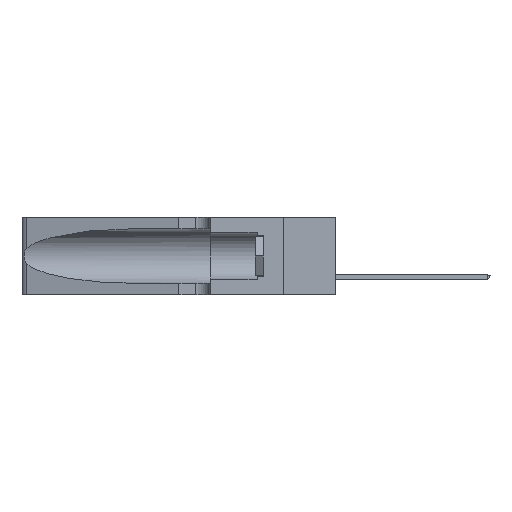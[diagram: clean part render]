
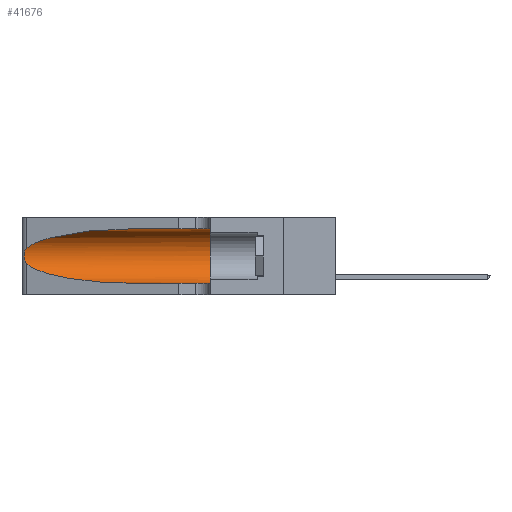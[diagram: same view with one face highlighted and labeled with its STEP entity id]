
A CAD part, left-side view. The second image highlights one B-rep face of the part: STEP entity #41676.
In plain terms, the highlighted cylindrical face has radius 3.308 mm (diameter 6.617 mm), a partial arc.
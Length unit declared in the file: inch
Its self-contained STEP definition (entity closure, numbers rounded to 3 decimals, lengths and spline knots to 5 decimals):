
#267 = EDGE_CURVE ( 'NONE', #30644, #3857, #19084, .T. ) ;
#515 = DIRECTION ( 'NONE',  ( 0., -1., 0. ) ) ;
#668 = VERTEX_POINT ( 'NONE', #48309 ) ;
#839 = FACE_OUTER_BOUND ( 'NONE', #32992, .T. ) ;
#2141 = CARTESIAN_POINT ( 'NONE',  ( 0.25487, 1.22718, 0.22369 ) ) ;
#3857 = VERTEX_POINT ( 'NONE', #40287 ) ;
#4057 = CARTESIAN_POINT ( 'NONE',  ( 0.25639, 1.23186, 0.15144 ) ) ;
#4203 = CARTESIAN_POINT ( 'NONE',  ( 0.1305, 1.61858, 0.31525 ) ) ;
#6728 = CARTESIAN_POINT ( 'NONE',  ( 0.25487, 1.22718, 0.14631 ) ) ;
#7945 = ORIENTED_EDGE ( 'NONE', *, *, #267, .F. ) ;
#7976 = CARTESIAN_POINT ( 'NONE',  ( 0.25487, 1.22718, 0.14631 ) ) ;
#9112 = VECTOR ( 'NONE', #19098, 39.37008 ) ;
#9765 = VERTEX_POINT ( 'NONE', #10908 ) ;
#10325 = AXIS2_PLACEMENT_3D ( 'NONE', #36463, #41348, #26176 ) ;
#10908 = CARTESIAN_POINT ( 'NONE',  ( 0.1305, 0.72297, 0.05475 ) ) ;
#11114 = ORIENTED_EDGE ( 'NONE', *, *, #35171, .F. ) ;
#11608 = CARTESIAN_POINT ( 'NONE',  ( 0.25555, 1.22993, 0.14849 ) ) ;
#11765 = VERTEX_POINT ( 'NONE', #6728 ) ;
#12239 = CARTESIAN_POINT ( 'NONE',  ( 0.1305, 1.61858, 0.05475 ) ) ;
#14107 =( BOUNDED_CURVE ( )  B_SPLINE_CURVE ( 3, ( #21835, #33135, #43877, #25896 ),
 .UNSPECIFIED., .F., .T. ) 
 B_SPLINE_CURVE_WITH_KNOTS ( ( 4, 4 ),
 ( 3.44316, 4.71239 ),
 .UNSPECIFIED. ) 
 CURVE ( )  GEOMETRIC_REPRESENTATION_ITEM ( )  RATIONAL_B_SPLINE_CURVE ( ( 1., 0.87, 0.87, 1. ) ) 
 REPRESENTATION_ITEM ( '' )  );
#14346 = EDGE_CURVE ( 'NONE', #9765, #668, #22334, .T. ) ;
#14579 = CARTESIAN_POINT ( 'NONE',  ( 0.1305, 0.72297, 0.31525 ) ) ;
#14739 = CARTESIAN_POINT ( 'NONE',  ( 0.2373, 1.15595, 0.28018 ) ) ;
#14792 = ORIENTED_EDGE ( 'NONE', *, *, #20571, .T. ) ;
#18055 = CARTESIAN_POINT ( 'NONE',  ( 0.26075, 1.23896, 0.178 ) ) ;
#18987 = CARTESIAN_POINT ( 'NONE',  ( 0.1305, 0.72297, 0.31525 ) ) ;
#19084 = LINE ( 'NONE', #4203, #9112 ) ;
#19098 = DIRECTION ( 'NONE',  ( 0., -1., 0. ) ) ;
#20571 = EDGE_CURVE ( 'NONE', #45771, #11765, #40152, .T. ) ;
#21597 = EDGE_CURVE ( 'NONE', #11765, #9765, #14107, .T. ) ;
#21835 = CARTESIAN_POINT ( 'NONE',  ( 0.25487, 1.22718, 0.14631 ) ) ;
#22334 = LINE ( 'NONE', #12239, #46883 ) ;
#22443 = CARTESIAN_POINT ( 'NONE',  ( 0.26075, 1.23896, 0.19203 ) ) ;
#22528 = CYLINDRICAL_SURFACE ( 'NONE', #25223, 0.13025 ) ;
#22649 = ORIENTED_EDGE ( 'NONE', *, *, #48252, .T. ) ;
#22928 = DIRECTION ( 'NONE',  ( 0., -1., 0. ) ) ;
#25223 = AXIS2_PLACEMENT_3D ( 'NONE', #26382, #515, #26540 ) ;
#25896 = CARTESIAN_POINT ( 'NONE',  ( 0.1305, 0.72297, 0.05475 ) ) ;
#26176 = DIRECTION ( 'NONE',  ( 0., 0., 1. ) ) ;
#26382 = CARTESIAN_POINT ( 'NONE',  ( 0.1305, 1.61858, 0.185 ) ) ;
#26540 = DIRECTION ( 'NONE',  ( 0., 0., -1. ) ) ;
#28528 = CARTESIAN_POINT ( 'NONE',  ( 0.25639, 1.23184, 0.21858 ) ) ;
#29644 = CARTESIAN_POINT ( 'NONE',  ( 0.18966, 0.96281, 0.31525 ) ) ;
#30644 = VERTEX_POINT ( 'NONE', #18987 ) ;
#32992 = EDGE_LOOP ( 'NONE', ( #22649, #14792, #44568, #33121, #11114, #7945 ) ) ;
#33121 = ORIENTED_EDGE ( 'NONE', *, *, #14346, .T. ) ;
#33135 = CARTESIAN_POINT ( 'NONE',  ( 0.2373, 1.15595, 0.08982 ) ) ;
#35047 = CARTESIAN_POINT ( 'NONE',  ( 0.25555, 1.22994, 0.2215 ) ) ;
#35171 = EDGE_CURVE ( 'NONE', #3857, #668, #48111, .T. ) ;
#36463 = CARTESIAN_POINT ( 'NONE',  ( 0.1305, 0.35, 0.185 ) ) ;
#37130 = CARTESIAN_POINT ( 'NONE',  ( 0.25854, 1.2359, 0.20912 ) ) ;
#40152 = B_SPLINE_CURVE_WITH_KNOTS ( 'NONE', 3,
 ( #2141, #35047, #28528, #41059, #37130, #44327, #22443, #18055, #44170, #45414, #45114, #4057, #11608, #7976 ),
 .UNSPECIFIED., .F., .F.,
 ( 4, 2, 2, 2, 2, 2, 4 ),
 ( 0., 0.00027, 0.00053, 0.00107, 0.0016, 0.00187, 0.00214 ),
 .UNSPECIFIED. ) ;
#40287 = CARTESIAN_POINT ( 'NONE',  ( 0.1305, 0.35, 0.31525 ) ) ;
#40713 = CARTESIAN_POINT ( 'NONE',  ( 0.25487, 1.22718, 0.22369 ) ) ;
#41059 = CARTESIAN_POINT ( 'NONE',  ( 0.25787, 1.23484, 0.2124 ) ) ;
#41348 = DIRECTION ( 'NONE',  ( 0., 1., 0. ) ) ;
#41490 = CARTESIAN_POINT ( 'NONE',  ( 0.25487, 1.22718, 0.22369 ) ) ;
#41676 = ADVANCED_FACE ( 'NONE', ( #839 ), #22528, .F. ) ;
#43877 = CARTESIAN_POINT ( 'NONE',  ( 0.18966, 0.96281, 0.05475 ) ) ;
#44170 = CARTESIAN_POINT ( 'NONE',  ( 0.26017, 1.23833, 0.17102 ) ) ;
#44327 = CARTESIAN_POINT ( 'NONE',  ( 0.26018, 1.23835, 0.19895 ) ) ;
#44568 = ORIENTED_EDGE ( 'NONE', *, *, #21597, .T. ) ;
#45114 = CARTESIAN_POINT ( 'NONE',  ( 0.25789, 1.23486, 0.15765 ) ) ;
#45414 = CARTESIAN_POINT ( 'NONE',  ( 0.25856, 1.23593, 0.16098 ) ) ;
#45481 =( BOUNDED_CURVE ( )  B_SPLINE_CURVE ( 3, ( #14579, #29644, #14739, #40713 ),
 .UNSPECIFIED., .F., .F. ) 
 B_SPLINE_CURVE_WITH_KNOTS ( ( 4, 4 ),
 ( 1.5708, 2.84003 ),
 .UNSPECIFIED. ) 
 CURVE ( )  GEOMETRIC_REPRESENTATION_ITEM ( )  RATIONAL_B_SPLINE_CURVE ( ( 1., 0.87, 0.87, 1. ) ) 
 REPRESENTATION_ITEM ( '' )  );
#45771 = VERTEX_POINT ( 'NONE', #41490 ) ;
#46883 = VECTOR ( 'NONE', #22928, 39.37008 ) ;
#48111 = CIRCLE ( 'NONE', #10325, 0.13025 ) ;
#48252 = EDGE_CURVE ( 'NONE', #30644, #45771, #45481, .T. ) ;
#48309 = CARTESIAN_POINT ( 'NONE',  ( 0.1305, 0.35, 0.05475 ) ) ;
